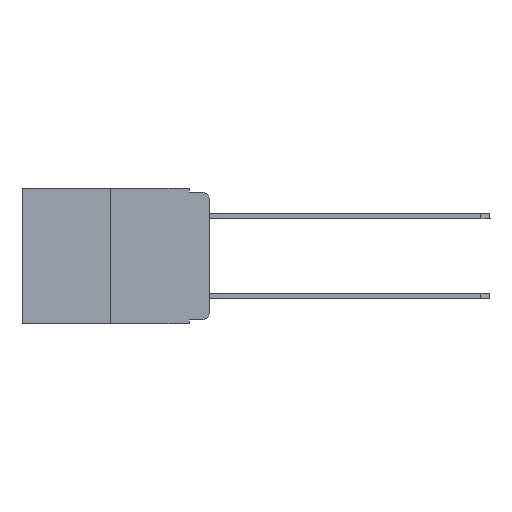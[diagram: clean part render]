
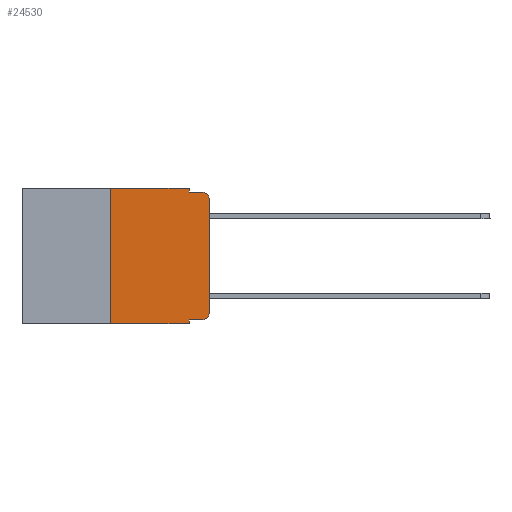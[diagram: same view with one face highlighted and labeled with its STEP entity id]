
A CAD part, left-side view. The second image highlights one B-rep face of the part: STEP entity #24530.
In plain terms, the highlighted planar face has unit normal (-1, 0, 0).
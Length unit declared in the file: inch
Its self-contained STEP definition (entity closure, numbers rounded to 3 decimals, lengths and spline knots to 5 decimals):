
#262 = DIRECTION ( 'NONE',  ( 0., 0., -1. ) ) ;
#484 = DIRECTION ( 'NONE',  ( 0., 0., -1. ) ) ;
#653 = VECTOR ( 'NONE', #10878, 39.37008 ) ;
#1369 = VERTEX_POINT ( 'NONE', #4160 ) ;
#1516 = VERTEX_POINT ( 'NONE', #20971 ) ;
#1777 = EDGE_CURVE ( 'NONE', #1516, #12604, #11195, .T. ) ;
#2710 = CARTESIAN_POINT ( 'NONE',  ( 0., 0.051, -0.333 ) ) ;
#3022 = DIRECTION ( 'NONE',  ( 0., -1., 0. ) ) ;
#3241 = DIRECTION ( 'NONE',  ( 0., 0., -1. ) ) ;
#3327 = FACE_OUTER_BOUND ( 'NONE', #13956, .T. ) ;
#3671 = CARTESIAN_POINT ( 'NONE',  ( 0., 0.02, -0.01 ) ) ;
#3684 = PLANE ( 'NONE',  #11965 ) ;
#3733 = VERTEX_POINT ( 'NONE', #19120 ) ;
#4142 = DIRECTION ( 'NONE',  ( -1., 0., 0. ) ) ;
#4160 = CARTESIAN_POINT ( 'NONE',  ( 0., 0.25, 0. ) ) ;
#4988 = CIRCLE ( 'NONE', #15097, 0.02 ) ;
#5105 = CARTESIAN_POINT ( 'NONE',  ( 0., 0.051, 0. ) ) ;
#5261 = CARTESIAN_POINT ( 'NONE',  ( 0., 0.051, 0. ) ) ;
#5829 = VECTOR ( 'NONE', #24676, 39.37008 ) ;
#5850 = EDGE_CURVE ( 'NONE', #6291, #15466, #7787, .T. ) ;
#5922 = EDGE_CURVE ( 'NONE', #7994, #3733, #17347, .T. ) ;
#5996 = EDGE_CURVE ( 'NONE', #7994, #1369, #20935, .T. ) ;
#6165 = VERTEX_POINT ( 'NONE', #17098 ) ;
#6291 = VERTEX_POINT ( 'NONE', #8655 ) ;
#6317 = CARTESIAN_POINT ( 'NONE',  ( 0., 0., -0.03 ) ) ;
#6318 = VERTEX_POINT ( 'NONE', #5105 ) ;
#6355 = EDGE_CURVE ( 'NONE', #6165, #3733, #22129, .T. ) ;
#7209 = VECTOR ( 'NONE', #22768, 39.37008 ) ;
#7655 = LINE ( 'NONE', #10856, #15105 ) ;
#7787 = LINE ( 'NONE', #10872, #21225 ) ;
#7994 = VERTEX_POINT ( 'NONE', #23847 ) ;
#8396 = CIRCLE ( 'NONE', #20493, 0.02 ) ;
#8465 = CARTESIAN_POINT ( 'NONE',  ( 0., 0.02, -0.313 ) ) ;
#8655 = CARTESIAN_POINT ( 'NONE',  ( 0., 0., -0.313 ) ) ;
#10081 = CARTESIAN_POINT ( 'NONE',  ( 0., 0.02, -0.03 ) ) ;
#10312 = DIRECTION ( 'NONE',  ( 0., -1., 0. ) ) ;
#10484 = ORIENTED_EDGE ( 'NONE', *, *, #12210, .T. ) ;
#10856 = CARTESIAN_POINT ( 'NONE',  ( 0., 0.051, 0. ) ) ;
#10872 = CARTESIAN_POINT ( 'NONE',  ( 0., 0., 0. ) ) ;
#10878 = DIRECTION ( 'NONE',  ( 0., 0., -1. ) ) ;
#11195 = LINE ( 'NONE', #14450, #17776 ) ;
#11813 = ORIENTED_EDGE ( 'NONE', *, *, #5922, .T. ) ;
#11859 = DIRECTION ( 'NONE',  ( -1., 0., 0. ) ) ;
#11965 = AXIS2_PLACEMENT_3D ( 'NONE', #24350, #15099, #18822 ) ;
#12210 = EDGE_CURVE ( 'NONE', #6165, #23090, #14343, .T. ) ;
#12604 = VERTEX_POINT ( 'NONE', #3671 ) ;
#13956 = EDGE_LOOP ( 'NONE', ( #19750, #16485, #20918, #15686, #14624, #19285, #11813, #18314, #10484, #22036 ) ) ;
#14343 = LINE ( 'NONE', #2710, #15236 ) ;
#14379 = EDGE_CURVE ( 'NONE', #23090, #6291, #8396, .T. ) ;
#14450 = CARTESIAN_POINT ( 'NONE',  ( 0., 0.051, -0.01 ) ) ;
#14624 = ORIENTED_EDGE ( 'NONE', *, *, #19464, .F. ) ;
#14994 = CARTESIAN_POINT ( 'NONE',  ( 0., 0.25, 0. ) ) ;
#15097 = AXIS2_PLACEMENT_3D ( 'NONE', #10081, #4142, #262 ) ;
#15099 = DIRECTION ( 'NONE',  ( 1., 0., 0. ) ) ;
#15105 = VECTOR ( 'NONE', #3241, 39.37008 ) ;
#15236 = VECTOR ( 'NONE', #10312, 39.37008 ) ;
#15466 = VERTEX_POINT ( 'NONE', #6317 ) ;
#15686 = ORIENTED_EDGE ( 'NONE', *, *, #18612, .F. ) ;
#16292 = DIRECTION ( 'NONE',  ( 0., 0., 1. ) ) ;
#16485 = ORIENTED_EDGE ( 'NONE', *, *, #20995, .T. ) ;
#16773 = DIRECTION ( 'NONE',  ( 0., -1., 0. ) ) ;
#16956 = CARTESIAN_POINT ( 'NONE',  ( 0., 0.473, 0. ) ) ;
#17061 = VECTOR ( 'NONE', #16773, 39.37008 ) ;
#17098 = CARTESIAN_POINT ( 'NONE',  ( 0., 0.051, -0.333 ) ) ;
#17347 = LINE ( 'NONE', #24721, #17061 ) ;
#17476 = LINE ( 'NONE', #16956, #5829 ) ;
#17776 = VECTOR ( 'NONE', #3022, 39.37008 ) ;
#18314 = ORIENTED_EDGE ( 'NONE', *, *, #6355, .F. ) ;
#18612 = EDGE_CURVE ( 'NONE', #6318, #1516, #7655, .T. ) ;
#18822 = DIRECTION ( 'NONE',  ( 0., 0., -1. ) ) ;
#19120 = CARTESIAN_POINT ( 'NONE',  ( 0., 0.051, -0.343 ) ) ;
#19285 = ORIENTED_EDGE ( 'NONE', *, *, #5996, .F. ) ;
#19464 = EDGE_CURVE ( 'NONE', #1369, #6318, #17476, .T. ) ;
#19750 = ORIENTED_EDGE ( 'NONE', *, *, #5850, .T. ) ;
#20493 = AXIS2_PLACEMENT_3D ( 'NONE', #8465, #11859, #484 ) ;
#20918 = ORIENTED_EDGE ( 'NONE', *, *, #1777, .F. ) ;
#20935 = LINE ( 'NONE', #14994, #7209 ) ;
#20971 = CARTESIAN_POINT ( 'NONE',  ( 0., 0.051, -0.01 ) ) ;
#20995 = EDGE_CURVE ( 'NONE', #15466, #12604, #4988, .T. ) ;
#21090 = CARTESIAN_POINT ( 'NONE',  ( 0., 0.02, -0.333 ) ) ;
#21225 = VECTOR ( 'NONE', #16292, 39.37008 ) ;
#22036 = ORIENTED_EDGE ( 'NONE', *, *, #14379, .T. ) ;
#22129 = LINE ( 'NONE', #5261, #653 ) ;
#22768 = DIRECTION ( 'NONE',  ( 0., 0., 1. ) ) ;
#23090 = VERTEX_POINT ( 'NONE', #21090 ) ;
#23847 = CARTESIAN_POINT ( 'NONE',  ( 0., 0.25, -0.343 ) ) ;
#24350 = CARTESIAN_POINT ( 'NONE',  ( 0., 0.473, 0. ) ) ;
#24530 = ADVANCED_FACE ( 'NONE', ( #3327 ), #3684, .F. ) ;
#24676 = DIRECTION ( 'NONE',  ( 0., -1., 0. ) ) ;
#24721 = CARTESIAN_POINT ( 'NONE',  ( 0., 0.473, -0.343 ) ) ;
